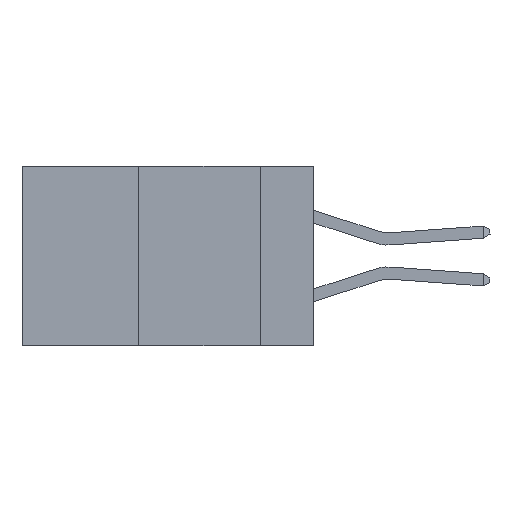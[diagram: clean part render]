
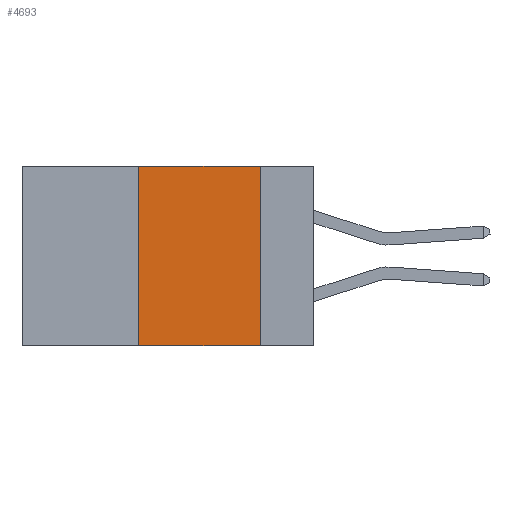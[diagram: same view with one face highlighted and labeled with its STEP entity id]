
A CAD part, left-side view. The second image highlights one B-rep face of the part: STEP entity #4693.
In plain terms, the highlighted planar face has unit normal (-1, 0, 0).
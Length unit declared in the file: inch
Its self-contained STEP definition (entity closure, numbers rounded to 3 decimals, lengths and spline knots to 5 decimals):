
#66 = LINE ( 'NONE', #11832, #3226 ) ;
#96 = PLANE ( 'NONE',  #10155 ) ;
#599 = CARTESIAN_POINT ( 'NONE',  ( 0., 0.36, 0. ) ) ;
#1386 = VECTOR ( 'NONE', #8680, 39.37008 ) ;
#1426 = VERTEX_POINT ( 'NONE', #7073 ) ;
#2274 = DIRECTION ( 'NONE',  ( 1., 0., 0. ) ) ;
#2429 = ORIENTED_EDGE ( 'NONE', *, *, #6863, .T. ) ;
#3167 = EDGE_CURVE ( 'NONE', #12086, #5064, #9006, .T. ) ;
#3226 = VECTOR ( 'NONE', #3940, 39.37008 ) ;
#3836 = CARTESIAN_POINT ( 'NONE',  ( 0., 0.11, -0.37 ) ) ;
#3940 = DIRECTION ( 'NONE',  ( 0., 0., 1. ) ) ;
#4693 = ADVANCED_FACE ( 'NONE', ( #13827 ), #96, .F. ) ;
#4793 = EDGE_CURVE ( 'NONE', #5064, #12898, #5684, .T. ) ;
#4984 = CARTESIAN_POINT ( 'NONE',  ( 0., 0.11, 0. ) ) ;
#5064 = VERTEX_POINT ( 'NONE', #4984 ) ;
#5684 = LINE ( 'NONE', #10370, #6769 ) ;
#5919 = VECTOR ( 'NONE', #6145, 39.37008 ) ;
#6145 = DIRECTION ( 'NONE',  ( 0., -1., 0. ) ) ;
#6373 = LINE ( 'NONE', #6377, #1386 ) ;
#6377 = CARTESIAN_POINT ( 'NONE',  ( 0., 0.6, -0.37 ) ) ;
#6381 = ORIENTED_EDGE ( 'NONE', *, *, #4793, .F. ) ;
#6769 = VECTOR ( 'NONE', #10426, 39.37008 ) ;
#6863 = EDGE_CURVE ( 'NONE', #1426, #12898, #6373, .T. ) ;
#6885 = DIRECTION ( 'NONE',  ( 0., 0., -1. ) ) ;
#7073 = CARTESIAN_POINT ( 'NONE',  ( 0., 0.36, -0.37 ) ) ;
#7623 = ORIENTED_EDGE ( 'NONE', *, *, #3167, .F. ) ;
#8173 = CARTESIAN_POINT ( 'NONE',  ( 0., 0.6, 0. ) ) ;
#8188 = ORIENTED_EDGE ( 'NONE', *, *, #10882, .F. ) ;
#8680 = DIRECTION ( 'NONE',  ( 0., -1., 0. ) ) ;
#9006 = LINE ( 'NONE', #10686, #5919 ) ;
#10155 = AXIS2_PLACEMENT_3D ( 'NONE', #8173, #2274, #6885 ) ;
#10370 = CARTESIAN_POINT ( 'NONE',  ( 0., 0.11, 0. ) ) ;
#10426 = DIRECTION ( 'NONE',  ( 0., 0., -1. ) ) ;
#10493 = EDGE_LOOP ( 'NONE', ( #6381, #7623, #8188, #2429 ) ) ;
#10686 = CARTESIAN_POINT ( 'NONE',  ( 0., 0.6, 0. ) ) ;
#10882 = EDGE_CURVE ( 'NONE', #1426, #12086, #66, .T. ) ;
#11832 = CARTESIAN_POINT ( 'NONE',  ( 0., 0.36, 0. ) ) ;
#12086 = VERTEX_POINT ( 'NONE', #599 ) ;
#12898 = VERTEX_POINT ( 'NONE', #3836 ) ;
#13827 = FACE_OUTER_BOUND ( 'NONE', #10493, .T. ) ;
